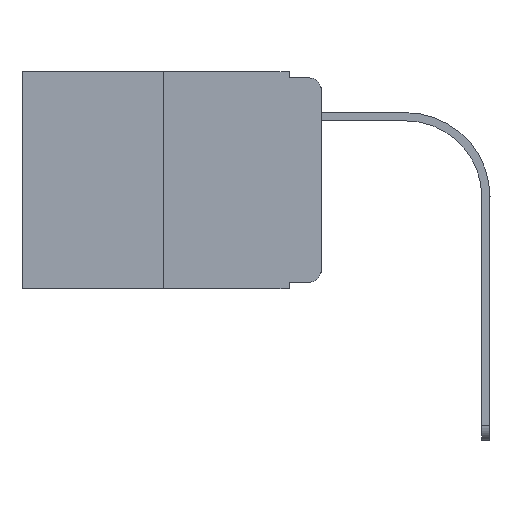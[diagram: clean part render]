
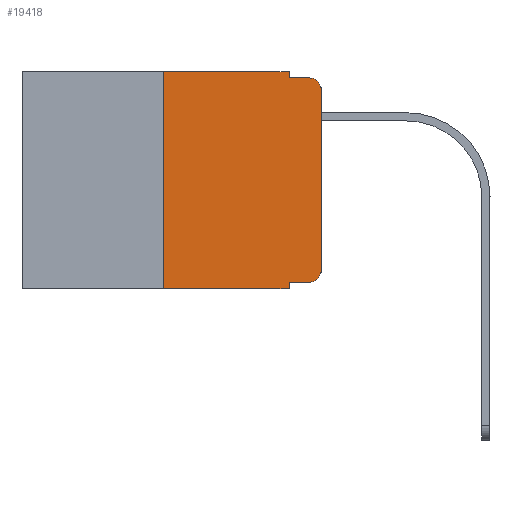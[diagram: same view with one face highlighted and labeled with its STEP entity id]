
A CAD part, left-side view. The second image highlights one B-rep face of the part: STEP entity #19418.
In plain terms, the highlighted planar face has unit normal (-1, 0, 0).
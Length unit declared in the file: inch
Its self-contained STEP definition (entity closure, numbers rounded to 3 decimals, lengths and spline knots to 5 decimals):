
#15 = CARTESIAN_POINT ( 'NONE',  ( 0., 0.051, 0. ) ) ;
#172 = CARTESIAN_POINT ( 'NONE',  ( 0., 0., -0.313 ) ) ;
#190 = ORIENTED_EDGE ( 'NONE', *, *, #18892, .T. ) ;
#254 = ORIENTED_EDGE ( 'NONE', *, *, #14283, .T. ) ;
#470 = LINE ( 'NONE', #13278, #5625 ) ;
#901 = ORIENTED_EDGE ( 'NONE', *, *, #7463, .T. ) ;
#962 = VERTEX_POINT ( 'NONE', #7264 ) ;
#1049 = ORIENTED_EDGE ( 'NONE', *, *, #16923, .F. ) ;
#1733 = ORIENTED_EDGE ( 'NONE', *, *, #19878, .F. ) ;
#2126 = CIRCLE ( 'NONE', #8843, 0.02 ) ;
#2351 = VECTOR ( 'NONE', #8012, 39.37008 ) ;
#2469 = VERTEX_POINT ( 'NONE', #3356 ) ;
#2843 = ORIENTED_EDGE ( 'NONE', *, *, #18640, .F. ) ;
#2999 = LINE ( 'NONE', #17450, #3246 ) ;
#3156 = DIRECTION ( 'NONE',  ( 0., 0., -1. ) ) ;
#3233 = ORIENTED_EDGE ( 'NONE', *, *, #10138, .F. ) ;
#3246 = VECTOR ( 'NONE', #16099, 39.37008 ) ;
#3356 = CARTESIAN_POINT ( 'NONE',  ( 0., 0.051, -0.333 ) ) ;
#3842 = PLANE ( 'NONE',  #8860 ) ;
#4122 = VECTOR ( 'NONE', #13286, 39.37008 ) ;
#4285 = DIRECTION ( 'NONE',  ( 0., 0., -1. ) ) ;
#4607 = ORIENTED_EDGE ( 'NONE', *, *, #4832, .T. ) ;
#4675 = AXIS2_PLACEMENT_3D ( 'NONE', #12809, #17721, #3156 ) ;
#4718 = ORIENTED_EDGE ( 'NONE', *, *, #5935, .T. ) ;
#4832 = EDGE_CURVE ( 'NONE', #10996, #17227, #2999, .T. ) ;
#5625 = VECTOR ( 'NONE', #14958, 39.37008 ) ;
#5638 = EDGE_CURVE ( 'NONE', #2469, #17111, #9427, .T. ) ;
#5935 = EDGE_CURVE ( 'NONE', #2469, #962, #470, .T. ) ;
#6074 = CARTESIAN_POINT ( 'NONE',  ( 0., 0.02, -0.01 ) ) ;
#6964 = CARTESIAN_POINT ( 'NONE',  ( 0., 0.02, -0.313 ) ) ;
#6978 = CIRCLE ( 'NONE', #4675, 0.02 ) ;
#7264 = CARTESIAN_POINT ( 'NONE',  ( 0., 0.02, -0.333 ) ) ;
#7463 = EDGE_CURVE ( 'NONE', #17227, #15336, #6978, .T. ) ;
#7655 = VECTOR ( 'NONE', #4285, 39.37008 ) ;
#7767 = CARTESIAN_POINT ( 'NONE',  ( 0., 0.051, 0. ) ) ;
#8012 = DIRECTION ( 'NONE',  ( 0., 0., -1. ) ) ;
#8843 = AXIS2_PLACEMENT_3D ( 'NONE', #6964, #13352, #11669 ) ;
#8860 = AXIS2_PLACEMENT_3D ( 'NONE', #10253, #12231, #14226 ) ;
#9027 = LINE ( 'NONE', #15302, #13430 ) ;
#9427 = LINE ( 'NONE', #7767, #7655 ) ;
#9510 = CARTESIAN_POINT ( 'NONE',  ( 0., 0.051, -0.343 ) ) ;
#9977 = VERTEX_POINT ( 'NONE', #12438 ) ;
#10138 = EDGE_CURVE ( 'NONE', #12719, #13600, #14111, .T. ) ;
#10253 = CARTESIAN_POINT ( 'NONE',  ( 0., 0.473, 0. ) ) ;
#10996 = VERTEX_POINT ( 'NONE', #172 ) ;
#11077 = EDGE_LOOP ( 'NONE', ( #4607, #901, #2843, #1733, #3233, #1049, #254, #18954, #4718, #190 ) ) ;
#11147 = CARTESIAN_POINT ( 'NONE',  ( 0., 0.051, 0. ) ) ;
#11289 = CARTESIAN_POINT ( 'NONE',  ( 0., 0.25, -0.343 ) ) ;
#11604 = LINE ( 'NONE', #19550, #4122 ) ;
#11669 = DIRECTION ( 'NONE',  ( 0., 0., -1. ) ) ;
#11927 = FACE_OUTER_BOUND ( 'NONE', #11077, .T. ) ;
#12155 = DIRECTION ( 'NONE',  ( 0., -1., 0. ) ) ;
#12231 = DIRECTION ( 'NONE',  ( 1., 0., 0. ) ) ;
#12438 = CARTESIAN_POINT ( 'NONE',  ( 0., 0.051, -0.01 ) ) ;
#12719 = VERTEX_POINT ( 'NONE', #15742 ) ;
#12749 = DIRECTION ( 'NONE',  ( 0., -1., 0. ) ) ;
#12809 = CARTESIAN_POINT ( 'NONE',  ( 0., 0.02, -0.03 ) ) ;
#13265 = VECTOR ( 'NONE', #12749, 39.37008 ) ;
#13278 = CARTESIAN_POINT ( 'NONE',  ( 0., 0.051, -0.333 ) ) ;
#13286 = DIRECTION ( 'NONE',  ( 0., 0., 1. ) ) ;
#13352 = DIRECTION ( 'NONE',  ( -1., 0., 0. ) ) ;
#13430 = VECTOR ( 'NONE', #12155, 39.37008 ) ;
#13600 = VERTEX_POINT ( 'NONE', #11147 ) ;
#14007 = DIRECTION ( 'NONE',  ( 0., -1., 0. ) ) ;
#14111 = LINE ( 'NONE', #20481, #13265 ) ;
#14226 = DIRECTION ( 'NONE',  ( 0., 0., -1. ) ) ;
#14283 = EDGE_CURVE ( 'NONE', #19558, #17111, #9027, .T. ) ;
#14958 = DIRECTION ( 'NONE',  ( 0., -1., 0. ) ) ;
#15302 = CARTESIAN_POINT ( 'NONE',  ( 0., 0.473, -0.343 ) ) ;
#15336 = VERTEX_POINT ( 'NONE', #6074 ) ;
#15742 = CARTESIAN_POINT ( 'NONE',  ( 0., 0.25, 0. ) ) ;
#16099 = DIRECTION ( 'NONE',  ( 0., 0., 1. ) ) ;
#16921 = LINE ( 'NONE', #18705, #17192 ) ;
#16923 = EDGE_CURVE ( 'NONE', #19558, #12719, #11604, .T. ) ;
#17111 = VERTEX_POINT ( 'NONE', #9510 ) ;
#17192 = VECTOR ( 'NONE', #14007, 39.37008 ) ;
#17207 = LINE ( 'NONE', #15, #2351 ) ;
#17227 = VERTEX_POINT ( 'NONE', #17666 ) ;
#17450 = CARTESIAN_POINT ( 'NONE',  ( 0., 0., 0. ) ) ;
#17666 = CARTESIAN_POINT ( 'NONE',  ( 0., 0., -0.03 ) ) ;
#17721 = DIRECTION ( 'NONE',  ( -1., 0., 0. ) ) ;
#18640 = EDGE_CURVE ( 'NONE', #9977, #15336, #16921, .T. ) ;
#18705 = CARTESIAN_POINT ( 'NONE',  ( 0., 0.051, -0.01 ) ) ;
#18892 = EDGE_CURVE ( 'NONE', #962, #10996, #2126, .T. ) ;
#18954 = ORIENTED_EDGE ( 'NONE', *, *, #5638, .F. ) ;
#19418 = ADVANCED_FACE ( 'NONE', ( #11927 ), #3842, .F. ) ;
#19550 = CARTESIAN_POINT ( 'NONE',  ( 0., 0.25, 0. ) ) ;
#19558 = VERTEX_POINT ( 'NONE', #11289 ) ;
#19878 = EDGE_CURVE ( 'NONE', #13600, #9977, #17207, .T. ) ;
#20481 = CARTESIAN_POINT ( 'NONE',  ( 0., 0.473, 0. ) ) ;
